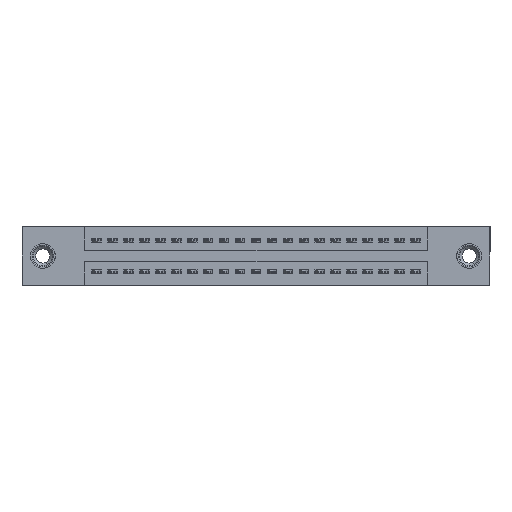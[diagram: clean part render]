
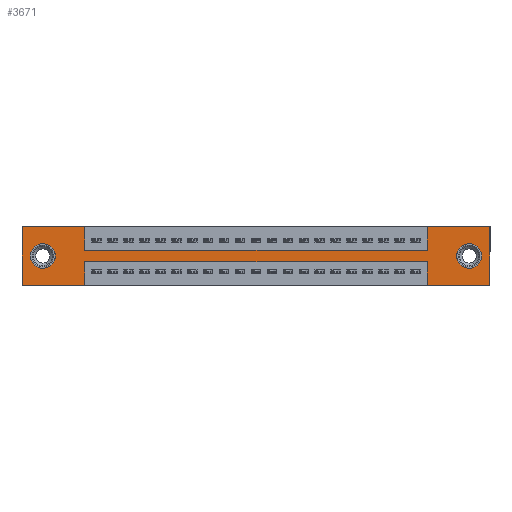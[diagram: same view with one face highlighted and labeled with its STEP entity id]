
A CAD part, front view. The second image highlights one B-rep face of the part: STEP entity #3671.
In plain terms, the highlighted planar face has unit normal (0, -1, 0).
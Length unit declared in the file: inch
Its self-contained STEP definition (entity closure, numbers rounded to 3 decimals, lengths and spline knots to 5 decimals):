
#102 = DIRECTION ( 'NONE',  ( 0., 0., 1. ) ) ;
#403 = VERTEX_POINT ( 'NONE', #14920 ) ;
#584 = CARTESIAN_POINT ( 'NONE',  ( 2.805, 0., -0.185 ) ) ;
#720 = VERTEX_POINT ( 'NONE', #15039 ) ;
#944 = CARTESIAN_POINT ( 'NONE',  ( 0., 0., -0.37 ) ) ;
#1287 = VERTEX_POINT ( 'NONE', #13743 ) ;
#1299 = CARTESIAN_POINT ( 'NONE',  ( 2.805, 0., -0.185 ) ) ;
#1308 = EDGE_CURVE ( 'NONE', #11314, #4311, #4126, .T. ) ;
#1317 = EDGE_LOOP ( 'NONE', ( #5704, #6237 ) ) ;
#1368 = EDGE_CURVE ( 'NONE', #3658, #1287, #3094, .T. ) ;
#1687 = CARTESIAN_POINT ( 'NONE',  ( 2.5425, 0., -0.37 ) ) ;
#1832 = DIRECTION ( 'NONE',  ( -1., 0., 0. ) ) ;
#2139 = CIRCLE ( 'NONE', #17893, 0.078 ) ;
#2259 = VECTOR ( 'NONE', #17963, 39.37008 ) ;
#2344 = DIRECTION ( 'NONE',  ( 0., 0., -1. ) ) ;
#2438 = CIRCLE ( 'NONE', #6327, 0.078 ) ;
#2559 = VECTOR ( 'NONE', #15524, 39.37008 ) ;
#2608 = DIRECTION ( 'NONE',  ( 0., 0., -1. ) ) ;
#3094 = LINE ( 'NONE', #16317, #2559 ) ;
#3281 = EDGE_CURVE ( 'NONE', #17771, #403, #11054, .T. ) ;
#3317 = EDGE_CURVE ( 'NONE', #15404, #17771, #10544, .T. ) ;
#3658 = VERTEX_POINT ( 'NONE', #12486 ) ;
#3671 = ADVANCED_FACE ( 'NONE', ( #3809, #20829, #4314 ), #19115, .T. ) ;
#3809 = FACE_BOUND ( 'NONE', #1317, .T. ) ;
#3831 = CARTESIAN_POINT ( 'NONE',  ( 0., 0., 0. ) ) ;
#4126 = CIRCLE ( 'NONE', #7189, 0.078 ) ;
#4164 = ORIENTED_EDGE ( 'NONE', *, *, #17493, .F. ) ;
#4311 = VERTEX_POINT ( 'NONE', #12672 ) ;
#4314 = FACE_OUTER_BOUND ( 'NONE', #5410, .T. ) ;
#4329 = DIRECTION ( 'NONE',  ( 0., 0., -1. ) ) ;
#4448 = VECTOR ( 'NONE', #18983, 39.37008 ) ;
#4572 = EDGE_CURVE ( 'NONE', #1287, #15404, #14832, .T. ) ;
#4828 = CARTESIAN_POINT ( 'NONE',  ( 0.3925, 0., -0.22 ) ) ;
#5361 = EDGE_CURVE ( 'NONE', #6103, #15860, #19014, .T. ) ;
#5410 = EDGE_LOOP ( 'NONE', ( #14264, #9937, #16946, #18613, #21387, #18706, #18677, #13851, #10536, #6995, #20665, #4164 ) ) ;
#5415 = AXIS2_PLACEMENT_3D ( 'NONE', #944, #14201, #4329 ) ;
#5482 = DIRECTION ( 'NONE',  ( 1., 0., 0. ) ) ;
#5704 = ORIENTED_EDGE ( 'NONE', *, *, #15742, .T. ) ;
#5761 = ORIENTED_EDGE ( 'NONE', *, *, #18059, .T. ) ;
#5872 = VECTOR ( 'NONE', #102, 39.37008 ) ;
#5882 = CARTESIAN_POINT ( 'NONE',  ( 0.3925, 0., -0.37 ) ) ;
#6103 = VERTEX_POINT ( 'NONE', #1687 ) ;
#6237 = ORIENTED_EDGE ( 'NONE', *, *, #1308, .T. ) ;
#6327 = AXIS2_PLACEMENT_3D ( 'NONE', #16405, #6547, #18062 ) ;
#6343 = EDGE_LOOP ( 'NONE', ( #11657, #5761 ) ) ;
#6454 = CARTESIAN_POINT ( 'NONE',  ( 2.5425, 0., 0. ) ) ;
#6547 = DIRECTION ( 'NONE',  ( 0., 1., 0. ) ) ;
#6760 = VERTEX_POINT ( 'NONE', #8061 ) ;
#6775 = DIRECTION ( 'NONE',  ( 1., 0., 0. ) ) ;
#6995 = ORIENTED_EDGE ( 'NONE', *, *, #11057, .F. ) ;
#7189 = AXIS2_PLACEMENT_3D ( 'NONE', #1299, #18695, #2608 ) ;
#7557 = CARTESIAN_POINT ( 'NONE',  ( 2.5425, 0., -0.22 ) ) ;
#7790 = CARTESIAN_POINT ( 'NONE',  ( 2.805, 0., -0.263 ) ) ;
#7997 = CARTESIAN_POINT ( 'NONE',  ( 2.935, 0., -0.37 ) ) ;
#8061 = CARTESIAN_POINT ( 'NONE',  ( 0.3925, 0., -0.37 ) ) ;
#8076 = CARTESIAN_POINT ( 'NONE',  ( 2.5425, 0., -0.15 ) ) ;
#8443 = CARTESIAN_POINT ( 'NONE',  ( 0., 0., -0.37 ) ) ;
#8700 = LINE ( 'NONE', #11319, #16937 ) ;
#8957 = DIRECTION ( 'NONE',  ( 0., 1., 0. ) ) ;
#9066 = EDGE_CURVE ( 'NONE', #12520, #6760, #13726, .T. ) ;
#9378 = CARTESIAN_POINT ( 'NONE',  ( 2.935, 0., 0. ) ) ;
#9758 = CARTESIAN_POINT ( 'NONE',  ( 0.3925, 0., -0.15 ) ) ;
#9877 = LINE ( 'NONE', #9378, #18116 ) ;
#9937 = ORIENTED_EDGE ( 'NONE', *, *, #17368, .F. ) ;
#10135 = LINE ( 'NONE', #3831, #13992 ) ;
#10364 = CARTESIAN_POINT ( 'NONE',  ( 0., 0., 0. ) ) ;
#10482 = VECTOR ( 'NONE', #6775, 39.37008 ) ;
#10515 = CARTESIAN_POINT ( 'NONE',  ( 0.3925, 0., -0.22 ) ) ;
#10536 = ORIENTED_EDGE ( 'NONE', *, *, #1368, .F. ) ;
#10544 = LINE ( 'NONE', #6454, #14375 ) ;
#11054 = LINE ( 'NONE', #16321, #2259 ) ;
#11057 = EDGE_CURVE ( 'NONE', #20664, #3658, #10135, .T. ) ;
#11303 = EDGE_CURVE ( 'NONE', #403, #20381, #9877, .T. ) ;
#11314 = VERTEX_POINT ( 'NONE', #7790 ) ;
#11319 = CARTESIAN_POINT ( 'NONE',  ( 0., 0., -0.37 ) ) ;
#11509 = AXIS2_PLACEMENT_3D ( 'NONE', #584, #12226, #2344 ) ;
#11657 = ORIENTED_EDGE ( 'NONE', *, *, #17021, .T. ) ;
#11695 = CARTESIAN_POINT ( 'NONE',  ( 2.5425, 0., -0.37 ) ) ;
#12226 = DIRECTION ( 'NONE',  ( 0., 1., 0. ) ) ;
#12486 = CARTESIAN_POINT ( 'NONE',  ( 0.3925, 0., 0. ) ) ;
#12520 = VERTEX_POINT ( 'NONE', #10515 ) ;
#12575 = DIRECTION ( 'NONE',  ( 0., 0., 1. ) ) ;
#12672 = CARTESIAN_POINT ( 'NONE',  ( 2.805, 0., -0.107 ) ) ;
#13299 = VECTOR ( 'NONE', #1832, 39.37008 ) ;
#13726 = LINE ( 'NONE', #5882, #4448 ) ;
#13743 = CARTESIAN_POINT ( 'NONE',  ( 0.3925, 0., -0.15 ) ) ;
#13796 = VERTEX_POINT ( 'NONE', #20321 ) ;
#13824 = LINE ( 'NONE', #8443, #13299 ) ;
#13851 = ORIENTED_EDGE ( 'NONE', *, *, #4572, .F. ) ;
#13992 = VECTOR ( 'NONE', #5482, 39.37008 ) ;
#14201 = DIRECTION ( 'NONE',  ( 0., -1., 0. ) ) ;
#14221 = CARTESIAN_POINT ( 'NONE',  ( 0., 0., 0. ) ) ;
#14264 = ORIENTED_EDGE ( 'NONE', *, *, #9066, .F. ) ;
#14375 = VECTOR ( 'NONE', #16390, 39.37008 ) ;
#14683 = DIRECTION ( 'NONE',  ( -1., 0., 0. ) ) ;
#14692 = VECTOR ( 'NONE', #12575, 39.37008 ) ;
#14832 = LINE ( 'NONE', #9758, #10482 ) ;
#14920 = CARTESIAN_POINT ( 'NONE',  ( 2.935, 0., 0. ) ) ;
#15039 = CARTESIAN_POINT ( 'NONE',  ( 0., 0., -0.37 ) ) ;
#15216 = LINE ( 'NONE', #14221, #14692 ) ;
#15404 = VERTEX_POINT ( 'NONE', #8076 ) ;
#15524 = DIRECTION ( 'NONE',  ( 0., 0., -1. ) ) ;
#15742 = EDGE_CURVE ( 'NONE', #4311, #11314, #17677, .T. ) ;
#15860 = VERTEX_POINT ( 'NONE', #7557 ) ;
#16317 = CARTESIAN_POINT ( 'NONE',  ( 0.3925, 0., 0. ) ) ;
#16321 = CARTESIAN_POINT ( 'NONE',  ( 0., 0., 0. ) ) ;
#16390 = DIRECTION ( 'NONE',  ( 0., 0., 1. ) ) ;
#16405 = CARTESIAN_POINT ( 'NONE',  ( 0.13, 0., -0.185 ) ) ;
#16422 = VECTOR ( 'NONE', #14683, 39.37008 ) ;
#16937 = VECTOR ( 'NONE', #21192, 39.37008 ) ;
#16946 = ORIENTED_EDGE ( 'NONE', *, *, #5361, .F. ) ;
#17021 = EDGE_CURVE ( 'NONE', #18583, #13796, #2139, .T. ) ;
#17313 = EDGE_CURVE ( 'NONE', #20381, #6103, #8700, .T. ) ;
#17368 = EDGE_CURVE ( 'NONE', #15860, #12520, #17454, .T. ) ;
#17430 = CARTESIAN_POINT ( 'NONE',  ( 2.5425, 0., 0. ) ) ;
#17454 = LINE ( 'NONE', #4828, #16422 ) ;
#17493 = EDGE_CURVE ( 'NONE', #6760, #720, #13824, .T. ) ;
#17677 = CIRCLE ( 'NONE', #11509, 0.078 ) ;
#17771 = VERTEX_POINT ( 'NONE', #17430 ) ;
#17893 = AXIS2_PLACEMENT_3D ( 'NONE', #18825, #8957, #20480 ) ;
#17963 = DIRECTION ( 'NONE',  ( 1., 0., 0. ) ) ;
#18059 = EDGE_CURVE ( 'NONE', #13796, #18583, #2438, .T. ) ;
#18062 = DIRECTION ( 'NONE',  ( 0., 0., 1. ) ) ;
#18116 = VECTOR ( 'NONE', #19239, 39.37008 ) ;
#18583 = VERTEX_POINT ( 'NONE', #19657 ) ;
#18613 = ORIENTED_EDGE ( 'NONE', *, *, #17313, .F. ) ;
#18677 = ORIENTED_EDGE ( 'NONE', *, *, #3317, .F. ) ;
#18695 = DIRECTION ( 'NONE',  ( 0., 1., 0. ) ) ;
#18706 = ORIENTED_EDGE ( 'NONE', *, *, #3281, .F. ) ;
#18825 = CARTESIAN_POINT ( 'NONE',  ( 0.13, 0., -0.185 ) ) ;
#18983 = DIRECTION ( 'NONE',  ( 0., 0., -1. ) ) ;
#19014 = LINE ( 'NONE', #11695, #5872 ) ;
#19115 = PLANE ( 'NONE',  #5415 ) ;
#19239 = DIRECTION ( 'NONE',  ( 0., 0., -1. ) ) ;
#19657 = CARTESIAN_POINT ( 'NONE',  ( 0.13, 0., -0.107 ) ) ;
#20321 = CARTESIAN_POINT ( 'NONE',  ( 0.13, 0., -0.263 ) ) ;
#20381 = VERTEX_POINT ( 'NONE', #7997 ) ;
#20480 = DIRECTION ( 'NONE',  ( 0., 0., 1. ) ) ;
#20664 = VERTEX_POINT ( 'NONE', #10364 ) ;
#20665 = ORIENTED_EDGE ( 'NONE', *, *, #20900, .F. ) ;
#20829 = FACE_BOUND ( 'NONE', #6343, .T. ) ;
#20900 = EDGE_CURVE ( 'NONE', #720, #20664, #15216, .T. ) ;
#21192 = DIRECTION ( 'NONE',  ( -1., 0., 0. ) ) ;
#21387 = ORIENTED_EDGE ( 'NONE', *, *, #11303, .F. ) ;
